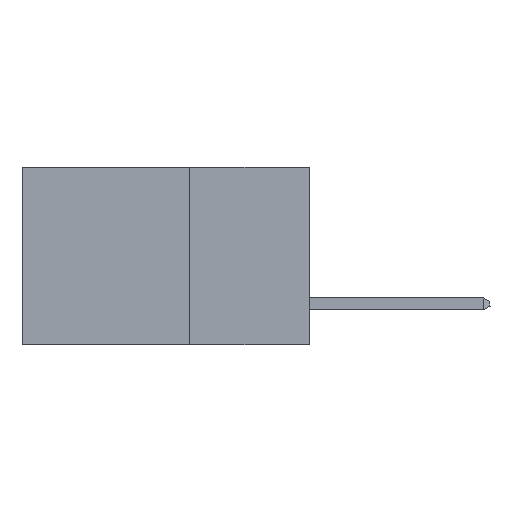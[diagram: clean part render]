
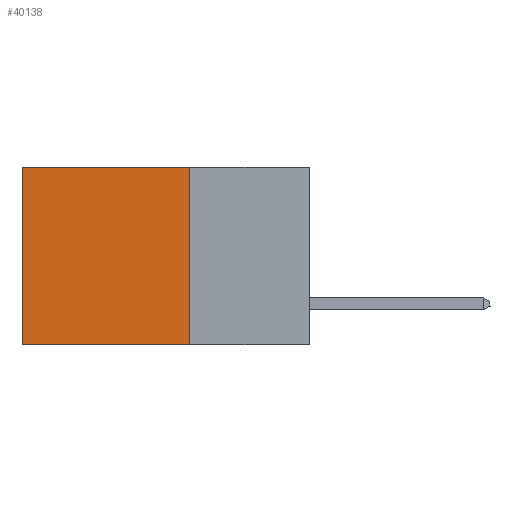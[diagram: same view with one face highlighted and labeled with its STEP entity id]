
A CAD part, left-side view. The second image highlights one B-rep face of the part: STEP entity #40138.
In plain terms, the highlighted planar face has unit normal (-1, 0, 0).
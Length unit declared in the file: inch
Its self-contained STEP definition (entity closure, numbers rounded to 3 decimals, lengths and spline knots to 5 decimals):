
#334 = VECTOR ( 'NONE', #21609, 39.37008 ) ;
#660 = DIRECTION ( 'NONE',  ( 0., 0., -1. ) ) ;
#2416 = CARTESIAN_POINT ( 'NONE',  ( 0.2875, 0.25, 0. ) ) ;
#2583 = VERTEX_POINT ( 'NONE', #24630 ) ;
#2952 = DIRECTION ( 'NONE',  ( 1., 0., 0. ) ) ;
#6023 = ORIENTED_EDGE ( 'NONE', *, *, #37118, .T. ) ;
#6382 = CARTESIAN_POINT ( 'NONE',  ( 0.2875, 0.25, -0.37 ) ) ;
#7157 = FACE_OUTER_BOUND ( 'NONE', #12938, .T. ) ;
#9429 = ORIENTED_EDGE ( 'NONE', *, *, #19280, .T. ) ;
#11470 = CARTESIAN_POINT ( 'NONE',  ( 0.2875, 0.25, 0. ) ) ;
#11528 = CARTESIAN_POINT ( 'NONE',  ( 0.2875, 0.6, 0. ) ) ;
#11649 = VECTOR ( 'NONE', #26153, 39.37008 ) ;
#11769 = VECTOR ( 'NONE', #660, 39.37008 ) ;
#12938 = EDGE_LOOP ( 'NONE', ( #9429, #25419, #20090, #6023 ) ) ;
#16346 = LINE ( 'NONE', #11528, #11649 ) ;
#19280 = EDGE_CURVE ( 'NONE', #22026, #2583, #16346, .T. ) ;
#19440 = AXIS2_PLACEMENT_3D ( 'NONE', #23025, #2952, #33563 ) ;
#19637 = VERTEX_POINT ( 'NONE', #29613 ) ;
#20054 = LINE ( 'NONE', #2416, #34163 ) ;
#20090 = ORIENTED_EDGE ( 'NONE', *, *, #24579, .F. ) ;
#20964 = CARTESIAN_POINT ( 'NONE',  ( 0.2875, 0.6, 0. ) ) ;
#21609 = DIRECTION ( 'NONE',  ( 0., 1., 0. ) ) ;
#21857 = LINE ( 'NONE', #24566, #334 ) ;
#22026 = VERTEX_POINT ( 'NONE', #20964 ) ;
#23025 = CARTESIAN_POINT ( 'NONE',  ( 0.2875, 0.25, 0. ) ) ;
#24566 = CARTESIAN_POINT ( 'NONE',  ( 0.2875, 0.25, -0.37 ) ) ;
#24579 = EDGE_CURVE ( 'NONE', #19637, #29515, #37412, .T. ) ;
#24630 = CARTESIAN_POINT ( 'NONE',  ( 0.2875, 0.6, -0.37 ) ) ;
#25419 = ORIENTED_EDGE ( 'NONE', *, *, #34379, .F. ) ;
#25605 = DIRECTION ( 'NONE',  ( 0., 1., 0. ) ) ;
#26153 = DIRECTION ( 'NONE',  ( 0., 0., -1. ) ) ;
#26677 = PLANE ( 'NONE',  #19440 ) ;
#29515 = VERTEX_POINT ( 'NONE', #6382 ) ;
#29613 = CARTESIAN_POINT ( 'NONE',  ( 0.2875, 0.25, 0. ) ) ;
#33563 = DIRECTION ( 'NONE',  ( 0., 0., -1. ) ) ;
#34163 = VECTOR ( 'NONE', #25605, 39.37008 ) ;
#34379 = EDGE_CURVE ( 'NONE', #29515, #2583, #21857, .T. ) ;
#37118 = EDGE_CURVE ( 'NONE', #19637, #22026, #20054, .T. ) ;
#37412 = LINE ( 'NONE', #11470, #11769 ) ;
#40138 = ADVANCED_FACE ( 'NONE', ( #7157 ), #26677, .F. ) ;
